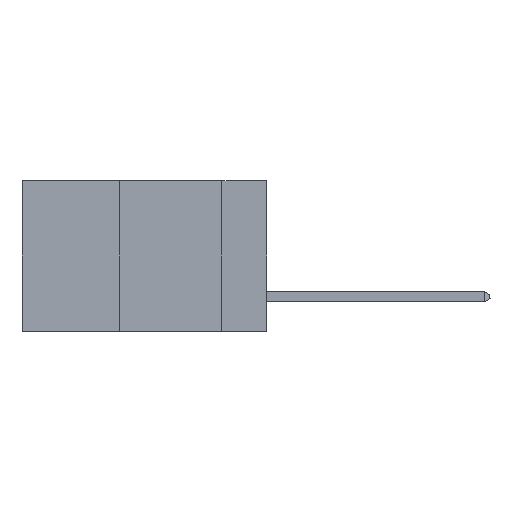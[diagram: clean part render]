
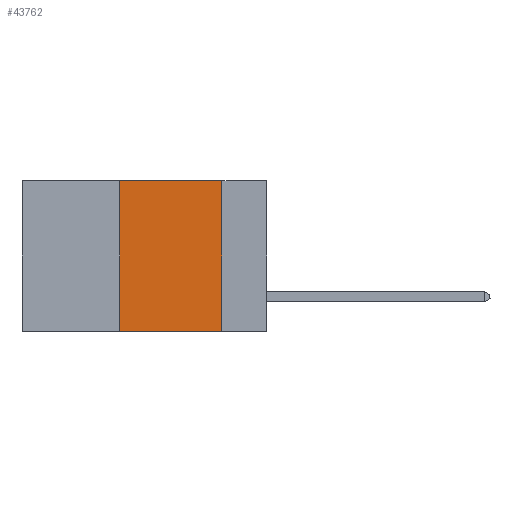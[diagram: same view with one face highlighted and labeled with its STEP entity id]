
A CAD part, left-side view. The second image highlights one B-rep face of the part: STEP entity #43762.
In plain terms, the highlighted planar face has unit normal (-1, 0, 0).
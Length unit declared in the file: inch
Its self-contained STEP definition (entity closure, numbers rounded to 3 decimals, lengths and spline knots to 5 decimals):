
#3817 = VERTEX_POINT ( 'NONE', #22990 ) ;
#5829 = VECTOR ( 'NONE', #22683, 39.37008 ) ;
#7327 = CARTESIAN_POINT ( 'NONE',  ( 0., 0.11, -0.37 ) ) ;
#8195 = AXIS2_PLACEMENT_3D ( 'NONE', #44324, #19014, #22998 ) ;
#8369 = CARTESIAN_POINT ( 'NONE',  ( 0., 0.6, 0. ) ) ;
#11146 = FACE_OUTER_BOUND ( 'NONE', #16633, .T. ) ;
#11376 = ORIENTED_EDGE ( 'NONE', *, *, #37817, .T. ) ;
#13703 = VERTEX_POINT ( 'NONE', #15417 ) ;
#13806 = CARTESIAN_POINT ( 'NONE',  ( 0., 0.36, 0. ) ) ;
#14280 = EDGE_CURVE ( 'NONE', #3817, #27494, #16069, .T. ) ;
#15417 = CARTESIAN_POINT ( 'NONE',  ( 0., 0.36, -0.37 ) ) ;
#16045 = VECTOR ( 'NONE', #20296, 39.37008 ) ;
#16069 = LINE ( 'NONE', #8369, #5829 ) ;
#16633 = EDGE_LOOP ( 'NONE', ( #44510, #31415, #34153, #11376 ) ) ;
#17190 = LINE ( 'NONE', #42390, #16045 ) ;
#17609 = DIRECTION ( 'NONE',  ( 0., 0., 1. ) ) ;
#19014 = DIRECTION ( 'NONE',  ( 1., 0., 0. ) ) ;
#20296 = DIRECTION ( 'NONE',  ( 0., -1., 0. ) ) ;
#20895 = DIRECTION ( 'NONE',  ( 0., 0., -1. ) ) ;
#21740 = EDGE_CURVE ( 'NONE', #27494, #27604, #32212, .T. ) ;
#22683 = DIRECTION ( 'NONE',  ( 0., -1., 0. ) ) ;
#22990 = CARTESIAN_POINT ( 'NONE',  ( 0., 0.36, 0. ) ) ;
#22998 = DIRECTION ( 'NONE',  ( 0., 0., -1. ) ) ;
#25980 = LINE ( 'NONE', #13806, #39628 ) ;
#27494 = VERTEX_POINT ( 'NONE', #28666 ) ;
#27604 = VERTEX_POINT ( 'NONE', #7327 ) ;
#28180 = EDGE_CURVE ( 'NONE', #13703, #3817, #25980, .T. ) ;
#28666 = CARTESIAN_POINT ( 'NONE',  ( 0., 0.11, 0. ) ) ;
#30311 = PLANE ( 'NONE',  #8195 ) ;
#31415 = ORIENTED_EDGE ( 'NONE', *, *, #14280, .F. ) ;
#32212 = LINE ( 'NONE', #46229, #33894 ) ;
#33894 = VECTOR ( 'NONE', #20895, 39.37008 ) ;
#34153 = ORIENTED_EDGE ( 'NONE', *, *, #28180, .F. ) ;
#37817 = EDGE_CURVE ( 'NONE', #13703, #27604, #17190, .T. ) ;
#39628 = VECTOR ( 'NONE', #17609, 39.37008 ) ;
#42390 = CARTESIAN_POINT ( 'NONE',  ( 0., 0.6, -0.37 ) ) ;
#43762 = ADVANCED_FACE ( 'NONE', ( #11146 ), #30311, .F. ) ;
#44324 = CARTESIAN_POINT ( 'NONE',  ( 0., 0.6, 0. ) ) ;
#44510 = ORIENTED_EDGE ( 'NONE', *, *, #21740, .F. ) ;
#46229 = CARTESIAN_POINT ( 'NONE',  ( 0., 0.11, 0. ) ) ;
